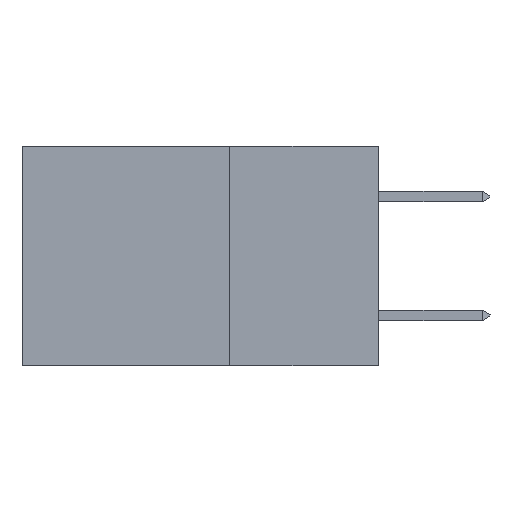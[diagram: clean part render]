
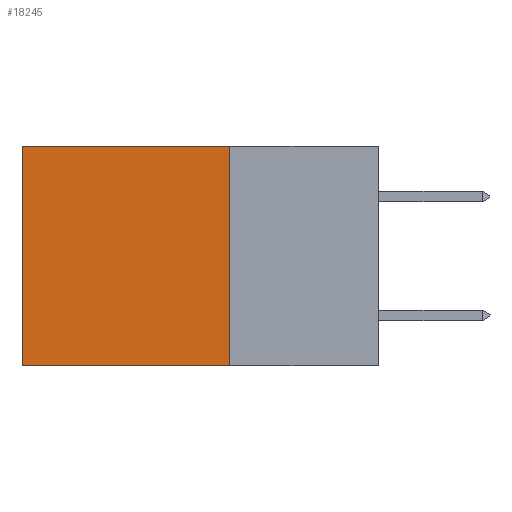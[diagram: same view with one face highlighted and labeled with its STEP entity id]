
A CAD part, left-side view. The second image highlights one B-rep face of the part: STEP entity #18245.
In plain terms, the highlighted planar face has unit normal (-1, 0, 0).
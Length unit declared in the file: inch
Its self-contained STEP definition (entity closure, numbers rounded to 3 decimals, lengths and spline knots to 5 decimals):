
#37 = DIRECTION ( 'NONE',  ( 0., 0., -1. ) ) ;
#66 = DIRECTION ( 'NONE',  ( 1., 0., 0. ) ) ;
#318 = VECTOR ( 'NONE', #10662, 39.37008 ) ;
#1522 = FACE_OUTER_BOUND ( 'NONE', #13712, .T. ) ;
#1547 = EDGE_CURVE ( 'NONE', #3068, #2920, #14876, .T. ) ;
#2068 = ORIENTED_EDGE ( 'NONE', *, *, #9575, .T. ) ;
#2920 = VERTEX_POINT ( 'NONE', #18806 ) ;
#3016 = CARTESIAN_POINT ( 'NONE',  ( 0.298, 0.6, 0. ) ) ;
#3068 = VERTEX_POINT ( 'NONE', #16638 ) ;
#3306 = LINE ( 'NONE', #8918, #10494 ) ;
#3659 = DIRECTION ( 'NONE',  ( 0., 1., 0. ) ) ;
#4299 = AXIS2_PLACEMENT_3D ( 'NONE', #14792, #66, #7322 ) ;
#5120 = EDGE_CURVE ( 'NONE', #18247, #2920, #3306, .T. ) ;
#5527 = ORIENTED_EDGE ( 'NONE', *, *, #5120, .T. ) ;
#6609 = CARTESIAN_POINT ( 'NONE',  ( 0.298, 0.25, 0. ) ) ;
#7322 = DIRECTION ( 'NONE',  ( 0., 0., -1. ) ) ;
#8383 = EDGE_CURVE ( 'NONE', #12194, #3068, #12901, .T. ) ;
#8918 = CARTESIAN_POINT ( 'NONE',  ( 0.298, 0.6, 0. ) ) ;
#9086 = CARTESIAN_POINT ( 'NONE',  ( 0.298, 0.25, 0. ) ) ;
#9575 = EDGE_CURVE ( 'NONE', #12194, #18247, #11908, .T. ) ;
#10494 = VECTOR ( 'NONE', #37, 39.37008 ) ;
#10662 = DIRECTION ( 'NONE',  ( 0., 1., 0. ) ) ;
#11908 = LINE ( 'NONE', #9086, #16741 ) ;
#12146 = ORIENTED_EDGE ( 'NONE', *, *, #1547, .F. ) ;
#12194 = VERTEX_POINT ( 'NONE', #6609 ) ;
#12392 = ORIENTED_EDGE ( 'NONE', *, *, #8383, .F. ) ;
#12901 = LINE ( 'NONE', #18511, #14040 ) ;
#13571 = CARTESIAN_POINT ( 'NONE',  ( 0.298, 0.25, -0.37 ) ) ;
#13712 = EDGE_LOOP ( 'NONE', ( #5527, #12146, #12392, #2068 ) ) ;
#14040 = VECTOR ( 'NONE', #18445, 39.37008 ) ;
#14792 = CARTESIAN_POINT ( 'NONE',  ( 0.298, 0.25, 0. ) ) ;
#14876 = LINE ( 'NONE', #13571, #318 ) ;
#16638 = CARTESIAN_POINT ( 'NONE',  ( 0.298, 0.25, -0.37 ) ) ;
#16741 = VECTOR ( 'NONE', #3659, 39.37008 ) ;
#17497 = PLANE ( 'NONE',  #4299 ) ;
#18245 = ADVANCED_FACE ( 'NONE', ( #1522 ), #17497, .F. ) ;
#18247 = VERTEX_POINT ( 'NONE', #3016 ) ;
#18445 = DIRECTION ( 'NONE',  ( 0., 0., -1. ) ) ;
#18511 = CARTESIAN_POINT ( 'NONE',  ( 0.298, 0.25, 0. ) ) ;
#18806 = CARTESIAN_POINT ( 'NONE',  ( 0.298, 0.6, -0.37 ) ) ;
